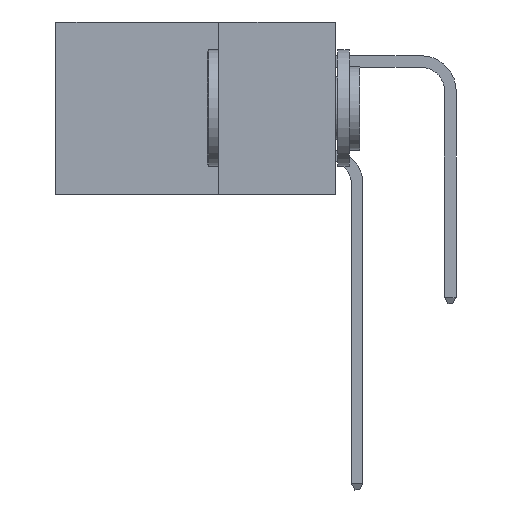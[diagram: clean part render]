
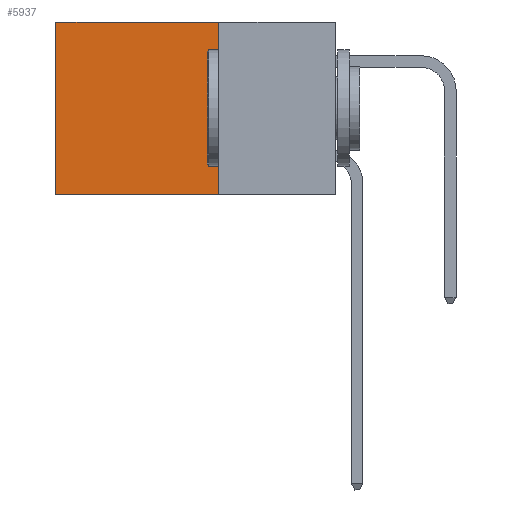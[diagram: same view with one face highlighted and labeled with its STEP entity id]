
A CAD part, left-side view. The second image highlights one B-rep face of the part: STEP entity #5937.
In plain terms, the highlighted planar face has unit normal (-1, 0, 0).
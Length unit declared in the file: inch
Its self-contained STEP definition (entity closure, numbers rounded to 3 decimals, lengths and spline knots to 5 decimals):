
#4 = EDGE_CURVE ( 'NONE', #12609, #14898, #4446, .T. ) ;
#897 = CARTESIAN_POINT ( 'NONE',  ( 0.2875, 0.6, 0. ) ) ;
#1222 = CARTESIAN_POINT ( 'NONE',  ( 0.2875, 0.25, -0.37 ) ) ;
#1865 = CARTESIAN_POINT ( 'NONE',  ( 0.2875, 0.25, 0. ) ) ;
#3510 = EDGE_CURVE ( 'NONE', #13725, #9500, #13715, .T. ) ;
#3609 = EDGE_CURVE ( 'NONE', #13725, #12609, #15928, .T. ) ;
#3679 = FACE_OUTER_BOUND ( 'NONE', #5957, .T. ) ;
#3866 = DIRECTION ( 'NONE',  ( 0., 0., -1. ) ) ;
#4446 = LINE ( 'NONE', #1222, #7534 ) ;
#4545 = CARTESIAN_POINT ( 'NONE',  ( 0.2875, 0.25, 0. ) ) ;
#5937 = ADVANCED_FACE ( 'NONE', ( #3679 ), #12858, .F. ) ;
#5957 = EDGE_LOOP ( 'NONE', ( #7950, #16715, #15057, #10017 ) ) ;
#7050 = CARTESIAN_POINT ( 'NONE',  ( 0.2875, 0.6, -0.37 ) ) ;
#7466 = CARTESIAN_POINT ( 'NONE',  ( 0.2875, 0.6, 0. ) ) ;
#7534 = VECTOR ( 'NONE', #9186, 39.37008 ) ;
#7950 = ORIENTED_EDGE ( 'NONE', *, *, #12589, .T. ) ;
#8338 = VECTOR ( 'NONE', #15090, 39.37008 ) ;
#8811 = DIRECTION ( 'NONE',  ( 0., 0., -1. ) ) ;
#9093 = LINE ( 'NONE', #897, #15887 ) ;
#9186 = DIRECTION ( 'NONE',  ( 0., 1., 0. ) ) ;
#9500 = VERTEX_POINT ( 'NONE', #7466 ) ;
#10017 = ORIENTED_EDGE ( 'NONE', *, *, #3510, .T. ) ;
#10198 = AXIS2_PLACEMENT_3D ( 'NONE', #16874, #10541, #3866 ) ;
#10541 = DIRECTION ( 'NONE',  ( 1., 0., 0. ) ) ;
#12589 = EDGE_CURVE ( 'NONE', #9500, #14898, #9093, .T. ) ;
#12609 = VERTEX_POINT ( 'NONE', #15532 ) ;
#12641 = VECTOR ( 'NONE', #12695, 39.37008 ) ;
#12695 = DIRECTION ( 'NONE',  ( 0., 0., -1. ) ) ;
#12858 = PLANE ( 'NONE',  #10198 ) ;
#13715 = LINE ( 'NONE', #4545, #8338 ) ;
#13725 = VERTEX_POINT ( 'NONE', #1865 ) ;
#14898 = VERTEX_POINT ( 'NONE', #7050 ) ;
#15057 = ORIENTED_EDGE ( 'NONE', *, *, #3609, .F. ) ;
#15090 = DIRECTION ( 'NONE',  ( 0., 1., 0. ) ) ;
#15292 = CARTESIAN_POINT ( 'NONE',  ( 0.2875, 0.25, 0. ) ) ;
#15532 = CARTESIAN_POINT ( 'NONE',  ( 0.2875, 0.25, -0.37 ) ) ;
#15887 = VECTOR ( 'NONE', #8811, 39.37008 ) ;
#15928 = LINE ( 'NONE', #15292, #12641 ) ;
#16715 = ORIENTED_EDGE ( 'NONE', *, *, #4, .F. ) ;
#16874 = CARTESIAN_POINT ( 'NONE',  ( 0.2875, 0.25, 0. ) ) ;
